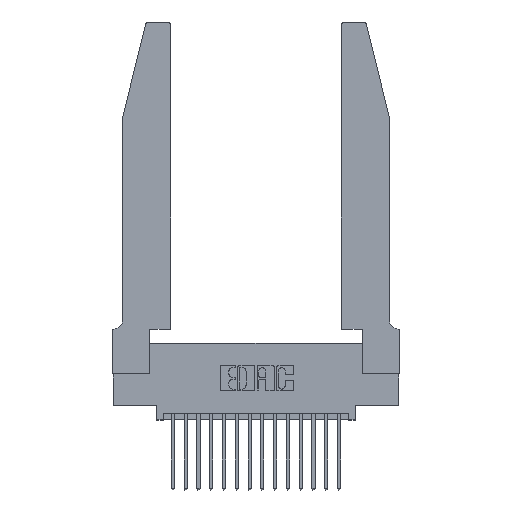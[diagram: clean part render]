
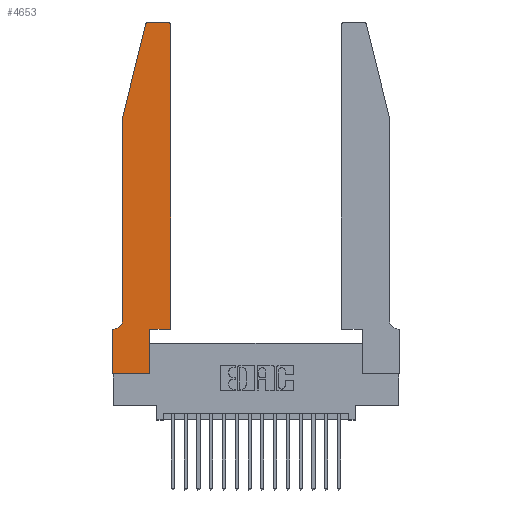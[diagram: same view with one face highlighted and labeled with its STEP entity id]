
A CAD part, top view. The second image highlights one B-rep face of the part: STEP entity #4653.
In plain terms, the highlighted planar face has unit normal (0, 0, 1).
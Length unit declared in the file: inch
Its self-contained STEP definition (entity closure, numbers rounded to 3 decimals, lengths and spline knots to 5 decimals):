
#51 = CARTESIAN_POINT ( 'NONE',  ( 0.0755, 2., 0.37 ) ) ;
#342 = CARTESIAN_POINT ( 'NONE',  ( 0.4505, 0.35, 0.37 ) ) ;
#1256 = VECTOR ( 'NONE', #18738, 39.37008 ) ;
#1921 = VERTEX_POINT ( 'NONE', #13464 ) ;
#1974 = CARTESIAN_POINT ( 'NONE',  ( 0.4505, 0.35, 0.37 ) ) ;
#2035 = DIRECTION ( 'NONE',  ( -0.239, -0.971, 0. ) ) ;
#2328 = EDGE_CURVE ( 'NONE', #1921, #16176, #2806, .T. ) ;
#2695 = VERTEX_POINT ( 'NONE', #10734 ) ;
#2703 = VERTEX_POINT ( 'NONE', #6144 ) ;
#2800 = AXIS2_PLACEMENT_3D ( 'NONE', #10674, #13652, #4654 ) ;
#2806 = LINE ( 'NONE', #17758, #11327 ) ;
#3061 = EDGE_CURVE ( 'NONE', #2703, #2695, #9396, .T. ) ;
#3630 = EDGE_CURVE ( 'NONE', #11130, #14097, #6513, .T. ) ;
#3868 = LINE ( 'NONE', #342, #1256 ) ;
#3869 = CARTESIAN_POINT ( 'NONE',  ( 0.2865, 0.35, 0.37 ) ) ;
#3892 = ORIENTED_EDGE ( 'NONE', *, *, #10583, .T. ) ;
#4108 = EDGE_CURVE ( 'NONE', #14455, #1921, #16985, .T. ) ;
#4162 = DIRECTION ( 'NONE',  ( 0., 0., -1. ) ) ;
#4264 = CIRCLE ( 'NONE', #10138, 0.03 ) ;
#4632 = VECTOR ( 'NONE', #16597, 39.37008 ) ;
#4653 = ADVANCED_FACE ( 'NONE', ( #8644 ), #6077, .T. ) ;
#4654 = DIRECTION ( 'NONE',  ( 1., 0., 0. ) ) ;
#5202 = DIRECTION ( 'NONE',  ( 1., 0., 0. ) ) ;
#5310 = DIRECTION ( 'NONE',  ( 0., -1., 0. ) ) ;
#5391 = DIRECTION ( 'NONE',  ( 0., 0., 1. ) ) ;
#5695 = DIRECTION ( 'NONE',  ( 0., 1., 0. ) ) ;
#5724 = ORIENTED_EDGE ( 'NONE', *, *, #4108, .T. ) ;
#5894 = LINE ( 'NONE', #18875, #7342 ) ;
#6077 = PLANE ( 'NONE',  #2800 ) ;
#6144 = CARTESIAN_POINT ( 'NONE',  ( 0.25487, 2.72718, 0.37 ) ) ;
#6323 = CARTESIAN_POINT ( 'NONE',  ( 0.284, 2.72, 0.37 ) ) ;
#6429 = CARTESIAN_POINT ( 'NONE',  ( 0.4505, 0.35, 0.37 ) ) ;
#6497 = DIRECTION ( 'NONE',  ( 0., 1., 0. ) ) ;
#6513 = LINE ( 'NONE', #6429, #17243 ) ;
#6518 = EDGE_CURVE ( 'NONE', #16176, #11130, #3868, .T. ) ;
#6588 = CARTESIAN_POINT ( 'NONE',  ( 0.4205, 2.72, 0.37 ) ) ;
#6684 = EDGE_CURVE ( 'NONE', #16459, #9463, #8595, .T. ) ;
#6825 = CARTESIAN_POINT ( 'NONE',  ( 0., 0.35, 0.37 ) ) ;
#6969 = CIRCLE ( 'NONE', #17686, 0.03 ) ;
#7082 = ORIENTED_EDGE ( 'NONE', *, *, #6518, .T. ) ;
#7342 = VECTOR ( 'NONE', #11108, 39.37008 ) ;
#7759 = VECTOR ( 'NONE', #7869, 39.37008 ) ;
#7869 = DIRECTION ( 'NONE',  ( -1., 0., 0. ) ) ;
#8190 = VECTOR ( 'NONE', #12063, 39.37008 ) ;
#8240 = VECTOR ( 'NONE', #2035, 39.37008 ) ;
#8515 = DIRECTION ( 'NONE',  ( 0., 0., 1. ) ) ;
#8540 = ORIENTED_EDGE ( 'NONE', *, *, #8604, .T. ) ;
#8595 = CIRCLE ( 'NONE', #10334, 0.07 ) ;
#8604 = EDGE_CURVE ( 'NONE', #9463, #8950, #14643, .T. ) ;
#8644 = FACE_OUTER_BOUND ( 'NONE', #18883, .T. ) ;
#8678 = CARTESIAN_POINT ( 'NONE',  ( 0.4205, 2.75, 0.37 ) ) ;
#8699 = ORIENTED_EDGE ( 'NONE', *, *, #2328, .T. ) ;
#8703 = ORIENTED_EDGE ( 'NONE', *, *, #3061, .T. ) ;
#8889 = CARTESIAN_POINT ( 'NONE',  ( 0., 0., 0.37 ) ) ;
#8950 = VERTEX_POINT ( 'NONE', #6825 ) ;
#9101 = CARTESIAN_POINT ( 'NONE',  ( 0.284, 2.75, 0.37 ) ) ;
#9396 = LINE ( 'NONE', #14272, #8240 ) ;
#9463 = VERTEX_POINT ( 'NONE', #17137 ) ;
#9689 = CARTESIAN_POINT ( 'NONE',  ( 0., 0., 0.37 ) ) ;
#9896 = ORIENTED_EDGE ( 'NONE', *, *, #13891, .T. ) ;
#10138 = AXIS2_PLACEMENT_3D ( 'NONE', #6323, #8515, #5202 ) ;
#10226 = VERTEX_POINT ( 'NONE', #9101 ) ;
#10334 = AXIS2_PLACEMENT_3D ( 'NONE', #13130, #4162, #11683 ) ;
#10583 = EDGE_CURVE ( 'NONE', #8950, #14455, #16477, .T. ) ;
#10674 = CARTESIAN_POINT ( 'NONE',  ( 0., 0.35, 0.37 ) ) ;
#10734 = CARTESIAN_POINT ( 'NONE',  ( 0.0755, 2., 0.37 ) ) ;
#10812 = ORIENTED_EDGE ( 'NONE', *, *, #6684, .T. ) ;
#11108 = DIRECTION ( 'NONE',  ( -1., 0., 0. ) ) ;
#11130 = VERTEX_POINT ( 'NONE', #1974 ) ;
#11327 = VECTOR ( 'NONE', #5695, 39.37008 ) ;
#11683 = DIRECTION ( 'NONE',  ( -1., 0., 0. ) ) ;
#11941 = ORIENTED_EDGE ( 'NONE', *, *, #3630, .T. ) ;
#11952 = LINE ( 'NONE', #51, #8190 ) ;
#12021 = VERTEX_POINT ( 'NONE', #8678 ) ;
#12063 = DIRECTION ( 'NONE',  ( 0., -1., 0. ) ) ;
#12817 = DIRECTION ( 'NONE',  ( 1., 0., 0. ) ) ;
#12993 = EDGE_CURVE ( 'NONE', #12021, #10226, #5894, .T. ) ;
#13130 = CARTESIAN_POINT ( 'NONE',  ( 0.0055, 0.42, 0.37 ) ) ;
#13440 = CARTESIAN_POINT ( 'NONE',  ( 0.0755, 0.42, 0.37 ) ) ;
#13464 = CARTESIAN_POINT ( 'NONE',  ( 0.2865, 0., 0.37 ) ) ;
#13652 = DIRECTION ( 'NONE',  ( 0., 0., 1. ) ) ;
#13819 = CARTESIAN_POINT ( 'NONE',  ( 0.0755, 0.35, 0.37 ) ) ;
#13891 = EDGE_CURVE ( 'NONE', #10226, #2703, #4264, .T. ) ;
#14097 = VERTEX_POINT ( 'NONE', #17014 ) ;
#14177 = ORIENTED_EDGE ( 'NONE', *, *, #18913, .T. ) ;
#14272 = CARTESIAN_POINT ( 'NONE',  ( 0.0755, 2., 0.37 ) ) ;
#14309 = CARTESIAN_POINT ( 'NONE',  ( 0., 0., 0.37 ) ) ;
#14320 = VECTOR ( 'NONE', #5310, 39.37008 ) ;
#14455 = VERTEX_POINT ( 'NONE', #14309 ) ;
#14643 = LINE ( 'NONE', #13819, #7759 ) ;
#14673 = EDGE_CURVE ( 'NONE', #14097, #12021, #6969, .T. ) ;
#16176 = VERTEX_POINT ( 'NONE', #3869 ) ;
#16459 = VERTEX_POINT ( 'NONE', #13440 ) ;
#16477 = LINE ( 'NONE', #9689, #14320 ) ;
#16597 = DIRECTION ( 'NONE',  ( 1., 0., 0. ) ) ;
#16985 = LINE ( 'NONE', #8889, #4632 ) ;
#17014 = CARTESIAN_POINT ( 'NONE',  ( 0.4505, 2.72, 0.37 ) ) ;
#17049 = ORIENTED_EDGE ( 'NONE', *, *, #12993, .T. ) ;
#17137 = CARTESIAN_POINT ( 'NONE',  ( 0.0055, 0.35, 0.37 ) ) ;
#17243 = VECTOR ( 'NONE', #6497, 39.37008 ) ;
#17686 = AXIS2_PLACEMENT_3D ( 'NONE', #6588, #5391, #12817 ) ;
#17758 = CARTESIAN_POINT ( 'NONE',  ( 0.2865, 0.35, 0.37 ) ) ;
#18738 = DIRECTION ( 'NONE',  ( 1., 0., 0. ) ) ;
#18875 = CARTESIAN_POINT ( 'NONE',  ( 0.2605, 2.75, 0.37 ) ) ;
#18883 = EDGE_LOOP ( 'NONE', ( #17049, #9896, #8703, #14177, #10812, #8540, #3892, #5724, #8699, #7082, #11941, #18987 ) ) ;
#18913 = EDGE_CURVE ( 'NONE', #2695, #16459, #11952, .T. ) ;
#18987 = ORIENTED_EDGE ( 'NONE', *, *, #14673, .T. ) ;
